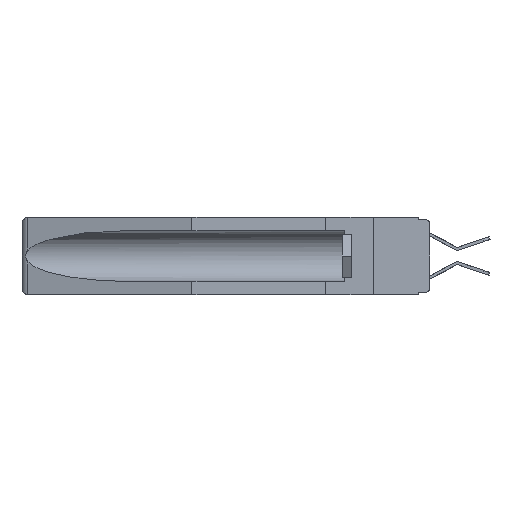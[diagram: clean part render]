
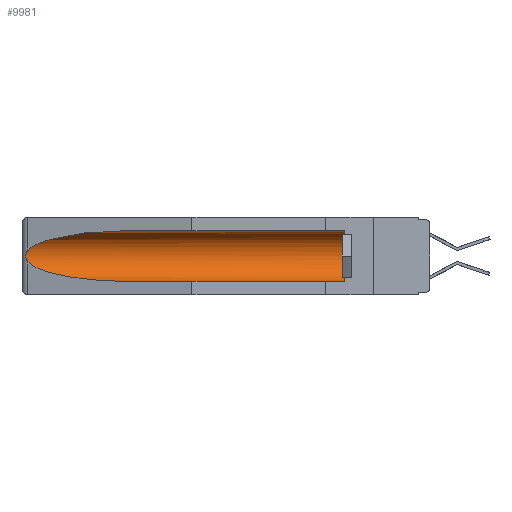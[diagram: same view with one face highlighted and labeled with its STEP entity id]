
A CAD part, left-side view. The second image highlights one B-rep face of the part: STEP entity #9981.
In plain terms, the highlighted cylindrical face has radius 2.857 mm (diameter 5.715 mm), a partial arc.
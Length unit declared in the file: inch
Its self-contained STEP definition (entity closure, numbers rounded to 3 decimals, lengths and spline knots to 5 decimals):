
#669 = EDGE_CURVE ( 'NONE', #3419, #11077, #21597, .T. ) ;
#911 = VERTEX_POINT ( 'NONE', #11927 ) ;
#1668 = VERTEX_POINT ( 'NONE', #20846 ) ;
#2081 = AXIS2_PLACEMENT_3D ( 'NONE', #3469, #12642, #24087 ) ;
#2139 = AXIS2_PLACEMENT_3D ( 'NONE', #5784, #22500, #16439 ) ;
#3419 = VERTEX_POINT ( 'NONE', #23047 ) ;
#3469 = CARTESIAN_POINT ( 'NONE',  ( 0.155, 0.126, -0.1715 ) ) ;
#3634 = CARTESIAN_POINT ( 'NONE',  ( 0.155, -0.30754, -0.284 ) ) ;
#3749 = DIRECTION ( 'NONE',  ( 0., 1., 0. ) ) ;
#3881 = LINE ( 'NONE', #3634, #7145 ) ;
#4664 =( BOUNDED_CURVE ( )  B_SPLINE_CURVE ( 3, ( #14909, #17120, #22314, #13420 ),
 .UNSPECIFIED., .F., .T. ) 
 B_SPLINE_CURVE_WITH_KNOTS ( ( 4, 4 ),
 ( 4.71239, 6.08839 ),
 .UNSPECIFIED. ) 
 CURVE ( )  GEOMETRIC_REPRESENTATION_ITEM ( )  RATIONAL_B_SPLINE_CURVE ( ( 1., 0.848, 0.848, 1. ) ) 
 REPRESENTATION_ITEM ( '' )  );
#5784 = CARTESIAN_POINT ( 'NONE',  ( 0.155, -0.30754, -0.1715 ) ) ;
#6847 = CARTESIAN_POINT ( 'NONE',  ( 0.155, 0.126, -0.284 ) ) ;
#7145 = VECTOR ( 'NONE', #20600, 39.37008 ) ;
#7238 = CARTESIAN_POINT ( 'NONE',  ( 0.26655, 1.53094, -0.18657 ) ) ;
#7327 = CARTESIAN_POINT ( 'NONE',  ( 0.155, 1.07973, -0.059 ) ) ;
#7353 = CARTESIAN_POINT ( 'NONE',  ( 0.26597, 1.52961, -0.15275 ) ) ;
#7635 = EDGE_LOOP ( 'NONE', ( #15577, #21042, #19116, #9088, #15125, #18040 ) ) ;
#8682 = CARTESIAN_POINT ( 'NONE',  ( 0.2675, 1.53308, -0.17534 ) ) ;
#9031 = VERTEX_POINT ( 'NONE', #6847 ) ;
#9088 = ORIENTED_EDGE ( 'NONE', *, *, #18050, .F. ) ;
#9981 = ADVANCED_FACE ( 'NONE', ( #15108 ), #13005, .F. ) ;
#10126 = CARTESIAN_POINT ( 'NONE',  ( 0.155, 1.07973, -0.284 ) ) ;
#10334 = CIRCLE ( 'NONE', #2081, 0.1125 ) ;
#11077 = VERTEX_POINT ( 'NONE', #10126 ) ;
#11927 = CARTESIAN_POINT ( 'NONE',  ( 0.155, 0.126, -0.059 ) ) ;
#12507 = CARTESIAN_POINT ( 'NONE',  ( 0.26537, 1.52718, -0.19328 ) ) ;
#12642 = DIRECTION ( 'NONE',  ( 0., -1., 0. ) ) ;
#12889 = CARTESIAN_POINT ( 'NONE',  ( 0.2675, 1.53308, -0.16763 ) ) ;
#12907 = EDGE_CURVE ( 'NONE', #9031, #911, #10334, .T. ) ;
#13005 = CYLINDRICAL_SURFACE ( 'NONE', #2139, 0.1125 ) ;
#13420 = CARTESIAN_POINT ( 'NONE',  ( 0.26537, 1.52718, -0.14972 ) ) ;
#14470 = CARTESIAN_POINT ( 'NONE',  ( 0.26654, 1.53092, -0.15636 ) ) ;
#14855 = CARTESIAN_POINT ( 'NONE',  ( 0.2673, 1.5327, -0.16383 ) ) ;
#14909 = CARTESIAN_POINT ( 'NONE',  ( 0.155, 1.07973, -0.059 ) ) ;
#15018 = CARTESIAN_POINT ( 'NONE',  ( 0.155, -0.30754, -0.059 ) ) ;
#15108 = FACE_OUTER_BOUND ( 'NONE', #7635, .T. ) ;
#15125 = ORIENTED_EDGE ( 'NONE', *, *, #12907, .T. ) ;
#15577 = ORIENTED_EDGE ( 'NONE', *, *, #23360, .T. ) ;
#15702 = EDGE_CURVE ( 'NONE', #911, #22724, #20572, .T. ) ;
#16439 = DIRECTION ( 'NONE',  ( 0., 0., 1. ) ) ;
#16460 = CARTESIAN_POINT ( 'NONE',  ( 0.155, 1.07973, -0.284 ) ) ;
#17120 = CARTESIAN_POINT ( 'NONE',  ( 0.21114, 1.30732, -0.059 ) ) ;
#18040 = ORIENTED_EDGE ( 'NONE', *, *, #15702, .T. ) ;
#18050 = EDGE_CURVE ( 'NONE', #9031, #11077, #3881, .T. ) ;
#18064 = CARTESIAN_POINT ( 'NONE',  ( 0.21114, 1.30732, -0.284 ) ) ;
#18406 = CARTESIAN_POINT ( 'NONE',  ( 0.26537, 1.52718, -0.14972 ) ) ;
#19116 = ORIENTED_EDGE ( 'NONE', *, *, #669, .T. ) ;
#19930 = CARTESIAN_POINT ( 'NONE',  ( 0.26537, 1.52718, -0.19328 ) ) ;
#20572 = LINE ( 'NONE', #15018, #21054 ) ;
#20600 = DIRECTION ( 'NONE',  ( 0., 1., 0. ) ) ;
#20846 = CARTESIAN_POINT ( 'NONE',  ( 0.26537, 1.52718, -0.14972 ) ) ;
#21042 = ORIENTED_EDGE ( 'NONE', *, *, #22371, .T. ) ;
#21054 = VECTOR ( 'NONE', #3749, 39.37008 ) ;
#21597 =( BOUNDED_CURVE ( )  B_SPLINE_CURVE ( 3, ( #19930, #23858, #18064, #16460 ),
 .UNSPECIFIED., .F., .T. ) 
 B_SPLINE_CURVE_WITH_KNOTS ( ( 4, 4 ),
 ( 0.1948, 1.5708 ),
 .UNSPECIFIED. ) 
 CURVE ( )  GEOMETRIC_REPRESENTATION_ITEM ( )  RATIONAL_B_SPLINE_CURVE ( ( 1., 0.848, 0.848, 1. ) ) 
 REPRESENTATION_ITEM ( '' )  );
#21731 = B_SPLINE_CURVE_WITH_KNOTS ( 'NONE', 3,
 ( #18406, #7353, #14470, #14855, #12889, #8682, #21988, #7238, #22368, #12507 ),
 .UNSPECIFIED., .F., .F.,
 ( 4, 2, 2, 2, 4 ),
 ( 0., 0.00029, 0.00058, 0.00087, 0.00117 ),
 .UNSPECIFIED. ) ;
#21988 = CARTESIAN_POINT ( 'NONE',  ( 0.2673, 1.53269, -0.17917 ) ) ;
#22314 = CARTESIAN_POINT ( 'NONE',  ( 0.25451, 1.48313, -0.09465 ) ) ;
#22368 = CARTESIAN_POINT ( 'NONE',  ( 0.26597, 1.5296, -0.19026 ) ) ;
#22371 = EDGE_CURVE ( 'NONE', #1668, #3419, #21731, .T. ) ;
#22500 = DIRECTION ( 'NONE',  ( 0., 1., 0. ) ) ;
#22724 = VERTEX_POINT ( 'NONE', #7327 ) ;
#23047 = CARTESIAN_POINT ( 'NONE',  ( 0.26537, 1.52718, -0.19328 ) ) ;
#23360 = EDGE_CURVE ( 'NONE', #22724, #1668, #4664, .T. ) ;
#23858 = CARTESIAN_POINT ( 'NONE',  ( 0.25451, 1.48313, -0.24835 ) ) ;
#24087 = DIRECTION ( 'NONE',  ( 0., 0., 1. ) ) ;
